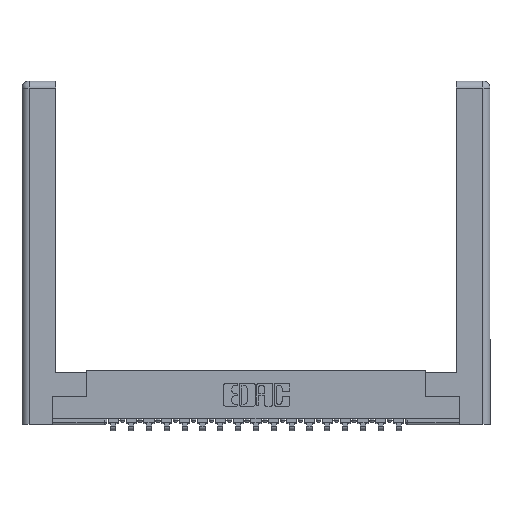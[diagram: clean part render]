
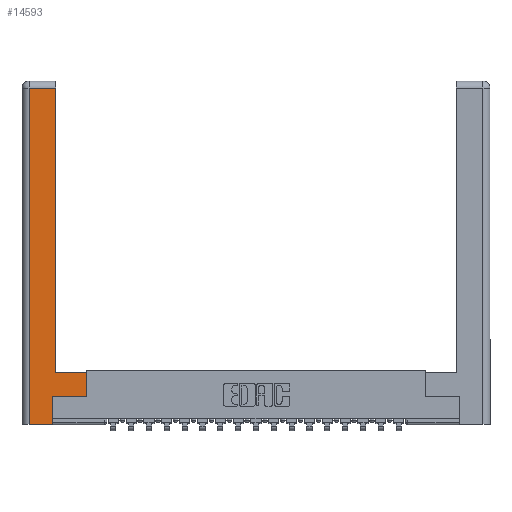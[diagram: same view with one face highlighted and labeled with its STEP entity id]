
A CAD part, top view. The second image highlights one B-rep face of the part: STEP entity #14593.
In plain terms, the highlighted planar face has unit normal (0, 0, 1).
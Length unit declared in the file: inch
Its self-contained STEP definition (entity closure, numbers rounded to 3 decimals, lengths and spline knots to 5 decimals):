
#41 = ORIENTED_EDGE ( 'NONE', *, *, #18545, .T. ) ;
#111 = LINE ( 'NONE', #5258, #11564 ) ;
#786 = DIRECTION ( 'NONE',  ( 0., 1., 0. ) ) ;
#1083 = ORIENTED_EDGE ( 'NONE', *, *, #13328, .T. ) ;
#1457 = VECTOR ( 'NONE', #6513, 39.37008 ) ;
#1732 = ORIENTED_EDGE ( 'NONE', *, *, #5730, .T. ) ;
#2150 = PLANE ( 'NONE',  #9340 ) ;
#2203 = CARTESIAN_POINT ( 'NONE',  ( 0.295, 2.94, 0. ) ) ;
#2756 = VERTEX_POINT ( 'NONE', #6104 ) ;
#3149 = ORIENTED_EDGE ( 'NONE', *, *, #14156, .T. ) ;
#3654 = VECTOR ( 'NONE', #9470, 39.37008 ) ;
#3729 = CARTESIAN_POINT ( 'NONE',  ( 0.565, 0.245, 0. ) ) ;
#3776 = DIRECTION ( 'NONE',  ( -1., 0., 0. ) ) ;
#4362 = EDGE_CURVE ( 'NONE', #12611, #19241, #8035, .T. ) ;
#4702 = VECTOR ( 'NONE', #786, 39.37008 ) ;
#4863 = VECTOR ( 'NONE', #6377, 39.37008 ) ;
#5258 = CARTESIAN_POINT ( 'NONE',  ( 0.0615, 2.94, 0. ) ) ;
#5659 = FACE_OUTER_BOUND ( 'NONE', #5838, .T. ) ;
#5707 = CARTESIAN_POINT ( 'NONE',  ( 0.0615, 2.94, 0. ) ) ;
#5730 = EDGE_CURVE ( 'NONE', #13923, #15695, #111, .T. ) ;
#5838 = EDGE_LOOP ( 'NONE', ( #12791, #1732, #7453, #19892, #3149, #41, #1083, #17112 ) ) ;
#6104 = CARTESIAN_POINT ( 'NONE',  ( 0.265, 0., 0. ) ) ;
#6377 = DIRECTION ( 'NONE',  ( 0., 1., 0. ) ) ;
#6513 = DIRECTION ( 'NONE',  ( 0., -1., 0. ) ) ;
#6631 = DIRECTION ( 'NONE',  ( 1., 0., 0. ) ) ;
#6659 = CARTESIAN_POINT ( 'NONE',  ( 0.0615, 0., 0. ) ) ;
#7085 = CARTESIAN_POINT ( 'NONE',  ( 0.0615, 0., 0. ) ) ;
#7453 = ORIENTED_EDGE ( 'NONE', *, *, #18406, .T. ) ;
#8035 = LINE ( 'NONE', #10694, #17503 ) ;
#8119 = CARTESIAN_POINT ( 'NONE',  ( 0.265, 0., 0. ) ) ;
#8249 = EDGE_CURVE ( 'NONE', #19241, #13923, #15543, .T. ) ;
#8554 = LINE ( 'NONE', #8119, #17493 ) ;
#9340 = AXIS2_PLACEMENT_3D ( 'NONE', #20101, #13529, #3776 ) ;
#9470 = DIRECTION ( 'NONE',  ( 0., 1., 0. ) ) ;
#9587 = DIRECTION ( 'NONE',  ( -1., 0., 0. ) ) ;
#9733 = CARTESIAN_POINT ( 'NONE',  ( 0.295, 3., 0. ) ) ;
#10295 = CARTESIAN_POINT ( 'NONE',  ( 0.565, 0.245, 0. ) ) ;
#10694 = CARTESIAN_POINT ( 'NONE',  ( 0.295, 0.45, 0. ) ) ;
#11564 = VECTOR ( 'NONE', #19954, 39.37008 ) ;
#11621 = LINE ( 'NONE', #3729, #20576 ) ;
#12087 = CARTESIAN_POINT ( 'NONE',  ( 0.565, 0.45, 0. ) ) ;
#12611 = VERTEX_POINT ( 'NONE', #16291 ) ;
#12791 = ORIENTED_EDGE ( 'NONE', *, *, #8249, .T. ) ;
#13328 = EDGE_CURVE ( 'NONE', #13987, #12611, #17717, .T. ) ;
#13529 = DIRECTION ( 'NONE',  ( 0., 0., -1. ) ) ;
#13923 = VERTEX_POINT ( 'NONE', #2203 ) ;
#13987 = VERTEX_POINT ( 'NONE', #10295 ) ;
#14156 = EDGE_CURVE ( 'NONE', #2756, #16412, #17417, .T. ) ;
#14593 = ADVANCED_FACE ( 'NONE', ( #5659 ), #2150, .F. ) ;
#15543 = LINE ( 'NONE', #9733, #4863 ) ;
#15597 = CARTESIAN_POINT ( 'NONE',  ( 0.265, 0.245, 0. ) ) ;
#15695 = VERTEX_POINT ( 'NONE', #5707 ) ;
#15833 = CARTESIAN_POINT ( 'NONE',  ( 0.265, 0.245, 0. ) ) ;
#16291 = CARTESIAN_POINT ( 'NONE',  ( 0.565, 0.45, 0. ) ) ;
#16412 = VERTEX_POINT ( 'NONE', #15597 ) ;
#16881 = CARTESIAN_POINT ( 'NONE',  ( 0.295, 0.45, 0. ) ) ;
#17112 = ORIENTED_EDGE ( 'NONE', *, *, #4362, .T. ) ;
#17417 = LINE ( 'NONE', #15833, #3654 ) ;
#17493 = VECTOR ( 'NONE', #6631, 39.37008 ) ;
#17503 = VECTOR ( 'NONE', #9587, 39.37008 ) ;
#17717 = LINE ( 'NONE', #12087, #4702 ) ;
#18165 = VERTEX_POINT ( 'NONE', #7085 ) ;
#18406 = EDGE_CURVE ( 'NONE', #15695, #18165, #20849, .T. ) ;
#18545 = EDGE_CURVE ( 'NONE', #16412, #13987, #11621, .T. ) ;
#19241 = VERTEX_POINT ( 'NONE', #16881 ) ;
#19892 = ORIENTED_EDGE ( 'NONE', *, *, #20497, .T. ) ;
#19954 = DIRECTION ( 'NONE',  ( -1., 0., 0. ) ) ;
#20052 = DIRECTION ( 'NONE',  ( 1., 0., 0. ) ) ;
#20101 = CARTESIAN_POINT ( 'NONE',  ( 0., 0., 0. ) ) ;
#20497 = EDGE_CURVE ( 'NONE', #18165, #2756, #8554, .T. ) ;
#20576 = VECTOR ( 'NONE', #20052, 39.37008 ) ;
#20849 = LINE ( 'NONE', #6659, #1457 ) ;
